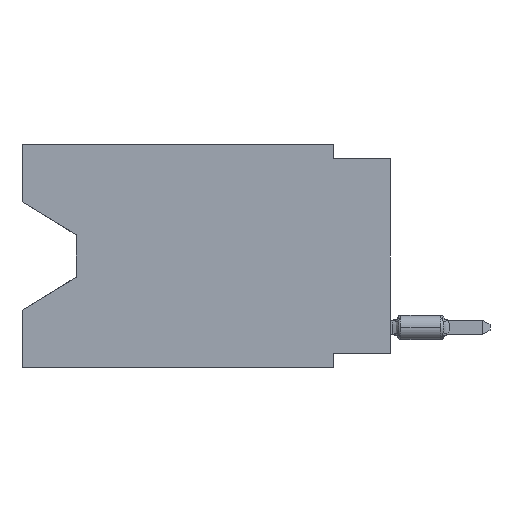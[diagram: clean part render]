
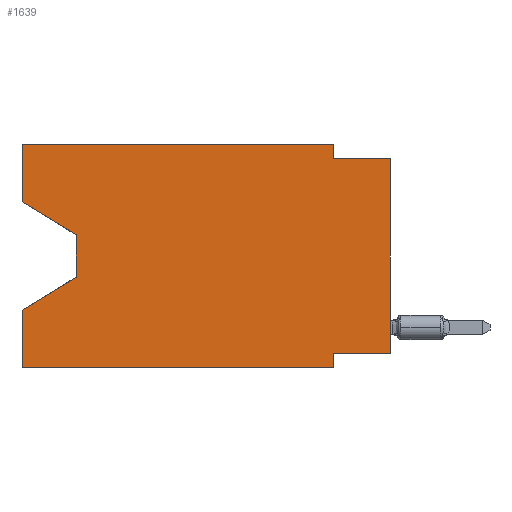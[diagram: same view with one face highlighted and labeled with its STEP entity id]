
A CAD part, left-side view. The second image highlights one B-rep face of the part: STEP entity #1639.
In plain terms, the highlighted planar face has unit normal (-1, 0, 0).
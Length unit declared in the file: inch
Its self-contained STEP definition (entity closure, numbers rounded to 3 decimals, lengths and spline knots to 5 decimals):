
#545 = CARTESIAN_POINT ( 'NONE',  ( 0., 0.645, -0.39 ) ) ;
#591 = CARTESIAN_POINT ( 'NONE',  ( 0., 0.645, 0. ) ) ;
#604 = CARTESIAN_POINT ( 'NONE',  ( 0., 0.645, -0.10025 ) ) ;
#664 = CARTESIAN_POINT ( 'NONE',  ( 0., 0.1, -0.39 ) ) ;
#675 = DIRECTION ( 'NONE',  ( 0., 0., 1. ) ) ;
#1596 = EDGE_CURVE ( 'NONE', #10331, #15374, #12317, .T. ) ;
#1639 = ADVANCED_FACE ( 'NONE', ( #15099 ), #19681, .F. ) ;
#1769 = VECTOR ( 'NONE', #5369, 39.37008 ) ;
#1788 = EDGE_CURVE ( 'NONE', #10039, #14405, #2254, .T. ) ;
#1865 = ORIENTED_EDGE ( 'NONE', *, *, #6958, .F. ) ;
#1872 = VECTOR ( 'NONE', #15059, 39.37008 ) ;
#2069 = LINE ( 'NONE', #14198, #18242 ) ;
#2254 = LINE ( 'NONE', #19258, #8568 ) ;
#2349 = DIRECTION ( 'NONE',  ( 0., -1., 0. ) ) ;
#2550 = ORIENTED_EDGE ( 'NONE', *, *, #1596, .T. ) ;
#2863 = CARTESIAN_POINT ( 'NONE',  ( 0., 0.55, -0.158 ) ) ;
#3045 = VERTEX_POINT ( 'NONE', #591 ) ;
#3077 = DIRECTION ( 'NONE',  ( 0., 0., 1. ) ) ;
#3309 = VECTOR ( 'NONE', #6730, 39.37008 ) ;
#3334 = VERTEX_POINT ( 'NONE', #18168 ) ;
#3415 = DIRECTION ( 'NONE',  ( 0., -1., 0. ) ) ;
#3908 = DIRECTION ( 'NONE',  ( 0., 1., 0. ) ) ;
#4647 = CARTESIAN_POINT ( 'NONE',  ( 0., 0.1, 0. ) ) ;
#4996 = CARTESIAN_POINT ( 'NONE',  ( 0., 0., -0.365 ) ) ;
#4998 = LINE ( 'NONE', #7636, #8625 ) ;
#5261 = VERTEX_POINT ( 'NONE', #14124 ) ;
#5369 = DIRECTION ( 'NONE',  ( 0., 0., -1. ) ) ;
#5466 = CARTESIAN_POINT ( 'NONE',  ( 0., 0.1, -0.025 ) ) ;
#5779 = DIRECTION ( 'NONE',  ( 0., 0.855, -0.519 ) ) ;
#6035 = CARTESIAN_POINT ( 'NONE',  ( 0., 0.645, 0. ) ) ;
#6210 = EDGE_CURVE ( 'NONE', #12601, #18360, #9900, .T. ) ;
#6268 = LINE ( 'NONE', #604, #15311 ) ;
#6456 = CARTESIAN_POINT ( 'NONE',  ( 0., 0.55, -0.232 ) ) ;
#6710 = ORIENTED_EDGE ( 'NONE', *, *, #10142, .F. ) ;
#6730 = DIRECTION ( 'NONE',  ( 0., 0., -1. ) ) ;
#6958 = EDGE_CURVE ( 'NONE', #3334, #8631, #2069, .T. ) ;
#7193 = CARTESIAN_POINT ( 'NONE',  ( 0., 0.645, 0. ) ) ;
#7455 = CARTESIAN_POINT ( 'NONE',  ( 0., 0., 0. ) ) ;
#7636 = CARTESIAN_POINT ( 'NONE',  ( 0., 0.645, 0. ) ) ;
#7637 = EDGE_CURVE ( 'NONE', #12601, #14405, #10657, .T. ) ;
#7670 = CARTESIAN_POINT ( 'NONE',  ( 0., 0.55, -0.232 ) ) ;
#8568 = VECTOR ( 'NONE', #2349, 39.37008 ) ;
#8625 = VECTOR ( 'NONE', #12588, 39.37008 ) ;
#8631 = VERTEX_POINT ( 'NONE', #19139 ) ;
#9283 = EDGE_CURVE ( 'NONE', #18360, #13516, #11212, .T. ) ;
#9700 = LINE ( 'NONE', #545, #12773 ) ;
#9868 = CARTESIAN_POINT ( 'NONE',  ( 0., 0.1, 0. ) ) ;
#9900 = LINE ( 'NONE', #11392, #16317 ) ;
#10039 = VERTEX_POINT ( 'NONE', #5466 ) ;
#10100 = ORIENTED_EDGE ( 'NONE', *, *, #1788, .F. ) ;
#10142 = EDGE_CURVE ( 'NONE', #16875, #10039, #11361, .T. ) ;
#10331 = VERTEX_POINT ( 'NONE', #10854 ) ;
#10606 = EDGE_LOOP ( 'NONE', ( #12158, #2550, #13555, #1865, #17263, #11422, #16960, #17815, #10100, #6710, #15702, #16710 ) ) ;
#10657 = LINE ( 'NONE', #7455, #13810 ) ;
#10702 = EDGE_CURVE ( 'NONE', #3334, #13516, #9700, .T. ) ;
#10730 = EDGE_CURVE ( 'NONE', #5261, #3045, #4998, .T. ) ;
#10854 = CARTESIAN_POINT ( 'NONE',  ( 0., 0.55, -0.158 ) ) ;
#10917 = CARTESIAN_POINT ( 'NONE',  ( 0., 0.1, -0.365 ) ) ;
#11212 = LINE ( 'NONE', #664, #3309 ) ;
#11361 = LINE ( 'NONE', #9868, #1769 ) ;
#11392 = CARTESIAN_POINT ( 'NONE',  ( 0., 0., -0.365 ) ) ;
#11422 = ORIENTED_EDGE ( 'NONE', *, *, #9283, .F. ) ;
#12122 = DIRECTION ( 'NONE',  ( 1., 0., 0. ) ) ;
#12158 = ORIENTED_EDGE ( 'NONE', *, *, #17657, .T. ) ;
#12164 = LINE ( 'NONE', #7670, #17514 ) ;
#12317 = LINE ( 'NONE', #2863, #16533 ) ;
#12588 = DIRECTION ( 'NONE',  ( 0., 0., 1. ) ) ;
#12601 = VERTEX_POINT ( 'NONE', #4996 ) ;
#12773 = VECTOR ( 'NONE', #3415, 39.37008 ) ;
#13516 = VERTEX_POINT ( 'NONE', #15083 ) ;
#13555 = ORIENTED_EDGE ( 'NONE', *, *, #16419, .T. ) ;
#13810 = VECTOR ( 'NONE', #3077, 39.37008 ) ;
#13921 = EDGE_CURVE ( 'NONE', #3045, #16875, #14865, .T. ) ;
#14124 = CARTESIAN_POINT ( 'NONE',  ( 0., 0.645, -0.10025 ) ) ;
#14198 = CARTESIAN_POINT ( 'NONE',  ( 0., 0.645, 0. ) ) ;
#14302 = AXIS2_PLACEMENT_3D ( 'NONE', #6035, #12122, #18191 ) ;
#14405 = VERTEX_POINT ( 'NONE', #15132 ) ;
#14865 = LINE ( 'NONE', #7193, #1872 ) ;
#15001 = DIRECTION ( 'NONE',  ( 0., 0., -1. ) ) ;
#15059 = DIRECTION ( 'NONE',  ( 0., -1., 0. ) ) ;
#15083 = CARTESIAN_POINT ( 'NONE',  ( 0., 0.1, -0.39 ) ) ;
#15099 = FACE_OUTER_BOUND ( 'NONE', #10606, .T. ) ;
#15132 = CARTESIAN_POINT ( 'NONE',  ( 0., 0., -0.025 ) ) ;
#15311 = VECTOR ( 'NONE', #18610, 39.37008 ) ;
#15374 = VERTEX_POINT ( 'NONE', #6456 ) ;
#15702 = ORIENTED_EDGE ( 'NONE', *, *, #13921, .F. ) ;
#16317 = VECTOR ( 'NONE', #3908, 39.37008 ) ;
#16419 = EDGE_CURVE ( 'NONE', #15374, #8631, #12164, .T. ) ;
#16533 = VECTOR ( 'NONE', #15001, 39.37008 ) ;
#16710 = ORIENTED_EDGE ( 'NONE', *, *, #10730, .F. ) ;
#16875 = VERTEX_POINT ( 'NONE', #4647 ) ;
#16960 = ORIENTED_EDGE ( 'NONE', *, *, #6210, .F. ) ;
#17263 = ORIENTED_EDGE ( 'NONE', *, *, #10702, .T. ) ;
#17514 = VECTOR ( 'NONE', #5779, 39.37008 ) ;
#17657 = EDGE_CURVE ( 'NONE', #5261, #10331, #6268, .T. ) ;
#17815 = ORIENTED_EDGE ( 'NONE', *, *, #7637, .T. ) ;
#18168 = CARTESIAN_POINT ( 'NONE',  ( 0., 0.645, -0.39 ) ) ;
#18191 = DIRECTION ( 'NONE',  ( 0., 0., -1. ) ) ;
#18242 = VECTOR ( 'NONE', #675, 39.37008 ) ;
#18360 = VERTEX_POINT ( 'NONE', #10917 ) ;
#18610 = DIRECTION ( 'NONE',  ( 0., -0.855, -0.519 ) ) ;
#19139 = CARTESIAN_POINT ( 'NONE',  ( 0., 0.645, -0.28975 ) ) ;
#19258 = CARTESIAN_POINT ( 'NONE',  ( 0., 0., -0.025 ) ) ;
#19681 = PLANE ( 'NONE',  #14302 ) ;
